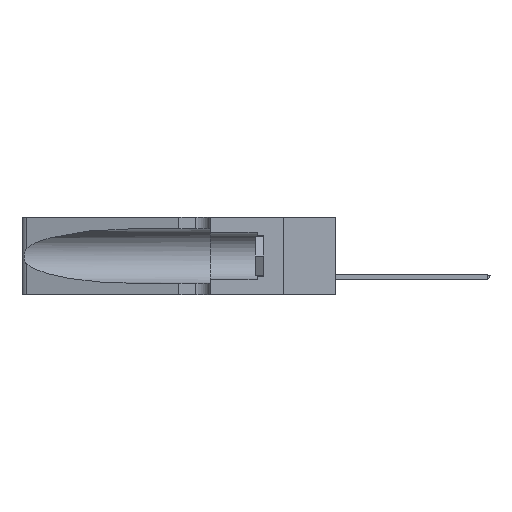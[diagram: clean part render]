
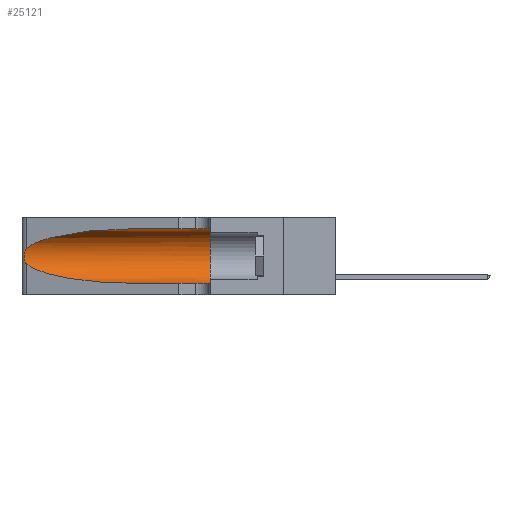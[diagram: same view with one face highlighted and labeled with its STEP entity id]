
A CAD part, left-side view. The second image highlights one B-rep face of the part: STEP entity #25121.
In plain terms, the highlighted cylindrical face has radius 3.308 mm (diameter 6.617 mm), a partial arc.
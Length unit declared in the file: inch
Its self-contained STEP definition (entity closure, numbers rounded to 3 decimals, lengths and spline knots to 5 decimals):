
#786 = CARTESIAN_POINT ( 'NONE',  ( 0.25787, 1.23484, 0.2124 ) ) ;
#1001 = CARTESIAN_POINT ( 'NONE',  ( 0.26017, 1.23833, 0.17102 ) ) ;
#1374 = DIRECTION ( 'NONE',  ( 0., -1., 0. ) ) ;
#1771 = DIRECTION ( 'NONE',  ( 0., -1., 0. ) ) ;
#1889 = EDGE_CURVE ( 'NONE', #17064, #18766, #8266, .T. ) ;
#1897 = CARTESIAN_POINT ( 'NONE',  ( 0.1305, 0.35, 0.185 ) ) ;
#2997 = ORIENTED_EDGE ( 'NONE', *, *, #8835, .T. ) ;
#3032 = CARTESIAN_POINT ( 'NONE',  ( 0.1305, 0.72297, 0.05475 ) ) ;
#3749 = CARTESIAN_POINT ( 'NONE',  ( 0.25487, 1.22718, 0.14631 ) ) ;
#3865 = DIRECTION ( 'NONE',  ( 0., 0., 1. ) ) ;
#4390 = VERTEX_POINT ( 'NONE', #5296 ) ;
#4489 = CARTESIAN_POINT ( 'NONE',  ( 0.1305, 1.61858, 0.185 ) ) ;
#5296 = CARTESIAN_POINT ( 'NONE',  ( 0.1305, 0.35, 0.31525 ) ) ;
#5602 = CARTESIAN_POINT ( 'NONE',  ( 0.25555, 1.22993, 0.14849 ) ) ;
#5807 = CARTESIAN_POINT ( 'NONE',  ( 0.25487, 1.22718, 0.22369 ) ) ;
#6424 = CARTESIAN_POINT ( 'NONE',  ( 0.25487, 1.22718, 0.22369 ) ) ;
#6902 = EDGE_CURVE ( 'NONE', #4390, #11764, #10936, .T. ) ;
#7989 = CARTESIAN_POINT ( 'NONE',  ( 0.25487, 1.22718, 0.14631 ) ) ;
#8266 =( BOUNDED_CURVE ( )  B_SPLINE_CURVE ( 3, ( #27022, #31015, #19738, #13694 ),
 .UNSPECIFIED., .F., .F. ) 
 B_SPLINE_CURVE_WITH_KNOTS ( ( 4, 4 ),
 ( 3.44316, 4.71239 ),
 .UNSPECIFIED. ) 
 CURVE ( )  GEOMETRIC_REPRESENTATION_ITEM ( )  RATIONAL_B_SPLINE_CURVE ( ( 1., 0.87, 0.87, 1. ) ) 
 REPRESENTATION_ITEM ( '' )  );
#8676 = VERTEX_POINT ( 'NONE', #6424 ) ;
#8835 = EDGE_CURVE ( 'NONE', #22433, #8676, #28344, .T. ) ;
#10010 = CARTESIAN_POINT ( 'NONE',  ( 0.25487, 1.22718, 0.22369 ) ) ;
#10489 = CARTESIAN_POINT ( 'NONE',  ( 0.25639, 1.23184, 0.21858 ) ) ;
#10713 = ORIENTED_EDGE ( 'NONE', *, *, #6902, .F. ) ;
#10936 = CIRCLE ( 'NONE', #19479, 0.13025 ) ;
#10944 = EDGE_CURVE ( 'NONE', #8676, #17064, #30641, .T. ) ;
#11138 = EDGE_LOOP ( 'NONE', ( #2997, #13231, #18993, #23474, #10713, #29783 ) ) ;
#11764 = VERTEX_POINT ( 'NONE', #26522 ) ;
#13231 = ORIENTED_EDGE ( 'NONE', *, *, #10944, .T. ) ;
#13354 = CARTESIAN_POINT ( 'NONE',  ( 0.1305, 1.61858, 0.31525 ) ) ;
#13665 = LINE ( 'NONE', #28818, #22287 ) ;
#13694 = CARTESIAN_POINT ( 'NONE',  ( 0.1305, 0.72297, 0.05475 ) ) ;
#15082 = CARTESIAN_POINT ( 'NONE',  ( 0.25555, 1.22994, 0.2215 ) ) ;
#15131 = CYLINDRICAL_SURFACE ( 'NONE', #23564, 0.13025 ) ;
#15301 = CARTESIAN_POINT ( 'NONE',  ( 0.26075, 1.23896, 0.19203 ) ) ;
#17064 = VERTEX_POINT ( 'NONE', #3749 ) ;
#17720 = CARTESIAN_POINT ( 'NONE',  ( 0.25856, 1.23593, 0.16098 ) ) ;
#18570 = DIRECTION ( 'NONE',  ( 0., 0., -1. ) ) ;
#18766 = VERTEX_POINT ( 'NONE', #3032 ) ;
#18993 = ORIENTED_EDGE ( 'NONE', *, *, #1889, .T. ) ;
#19341 = DIRECTION ( 'NONE',  ( 0., -1., 0. ) ) ;
#19479 = AXIS2_PLACEMENT_3D ( 'NONE', #1897, #20996, #3865 ) ;
#19738 = CARTESIAN_POINT ( 'NONE',  ( 0.18966, 0.96281, 0.05475 ) ) ;
#19897 = CARTESIAN_POINT ( 'NONE',  ( 0.25639, 1.23186, 0.15144 ) ) ;
#20233 = CARTESIAN_POINT ( 'NONE',  ( 0.25854, 1.2359, 0.20912 ) ) ;
#20791 = FACE_OUTER_BOUND ( 'NONE', #11138, .T. ) ;
#20996 = DIRECTION ( 'NONE',  ( 0., 1., 0. ) ) ;
#21953 = CARTESIAN_POINT ( 'NONE',  ( 0.18966, 0.96281, 0.31525 ) ) ;
#22287 = VECTOR ( 'NONE', #19341, 39.37008 ) ;
#22344 = CARTESIAN_POINT ( 'NONE',  ( 0.25789, 1.23486, 0.15765 ) ) ;
#22433 = VERTEX_POINT ( 'NONE', #25804 ) ;
#22682 = CARTESIAN_POINT ( 'NONE',  ( 0.26075, 1.23896, 0.178 ) ) ;
#23474 = ORIENTED_EDGE ( 'NONE', *, *, #25242, .T. ) ;
#23564 = AXIS2_PLACEMENT_3D ( 'NONE', #4489, #1771, #18570 ) ;
#25121 = ADVANCED_FACE ( 'NONE', ( #20791 ), #15131, .F. ) ;
#25242 = EDGE_CURVE ( 'NONE', #18766, #11764, #13665, .T. ) ;
#25466 = VECTOR ( 'NONE', #1374, 39.37008 ) ;
#25804 = CARTESIAN_POINT ( 'NONE',  ( 0.1305, 0.72297, 0.31525 ) ) ;
#26522 = CARTESIAN_POINT ( 'NONE',  ( 0.1305, 0.35, 0.05475 ) ) ;
#27022 = CARTESIAN_POINT ( 'NONE',  ( 0.25487, 1.22718, 0.14631 ) ) ;
#27348 = CARTESIAN_POINT ( 'NONE',  ( 0.26018, 1.23835, 0.19895 ) ) ;
#28344 =( BOUNDED_CURVE ( )  B_SPLINE_CURVE ( 3, ( #29505, #21953, #29609, #10010 ),
 .UNSPECIFIED., .F., .F. ) 
 B_SPLINE_CURVE_WITH_KNOTS ( ( 4, 4 ),
 ( 1.5708, 2.84003 ),
 .UNSPECIFIED. ) 
 CURVE ( )  GEOMETRIC_REPRESENTATION_ITEM ( )  RATIONAL_B_SPLINE_CURVE ( ( 1., 0.87, 0.87, 1. ) ) 
 REPRESENTATION_ITEM ( '' )  );
#28818 = CARTESIAN_POINT ( 'NONE',  ( 0.1305, 1.61858, 0.05475 ) ) ;
#29505 = CARTESIAN_POINT ( 'NONE',  ( 0.1305, 0.72297, 0.31525 ) ) ;
#29609 = CARTESIAN_POINT ( 'NONE',  ( 0.2373, 1.15595, 0.28018 ) ) ;
#29768 = EDGE_CURVE ( 'NONE', #22433, #4390, #31132, .T. ) ;
#29783 = ORIENTED_EDGE ( 'NONE', *, *, #29768, .F. ) ;
#30641 = B_SPLINE_CURVE_WITH_KNOTS ( 'NONE', 3,
 ( #5807, #15082, #10489, #786, #20233, #27348, #15301, #22682, #1001, #17720, #22344, #19897, #5602, #7989 ),
 .UNSPECIFIED., .F., .F.,
 ( 4, 2, 2, 2, 2, 2, 4 ),
 ( 0., 0.00027, 0.00053, 0.00107, 0.0016, 0.00187, 0.00214 ),
 .UNSPECIFIED. ) ;
#31015 = CARTESIAN_POINT ( 'NONE',  ( 0.2373, 1.15595, 0.08982 ) ) ;
#31132 = LINE ( 'NONE', #13354, #25466 ) ;
